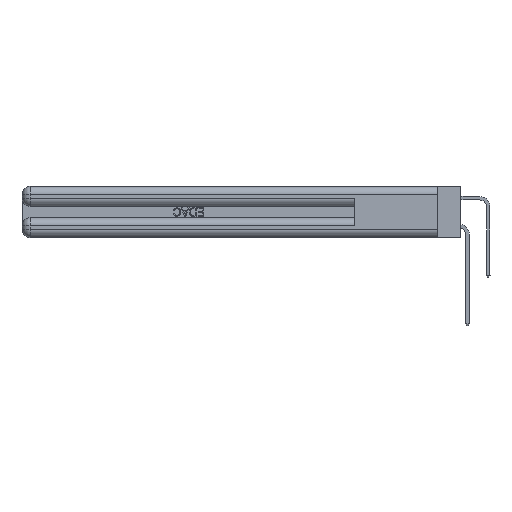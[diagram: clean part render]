
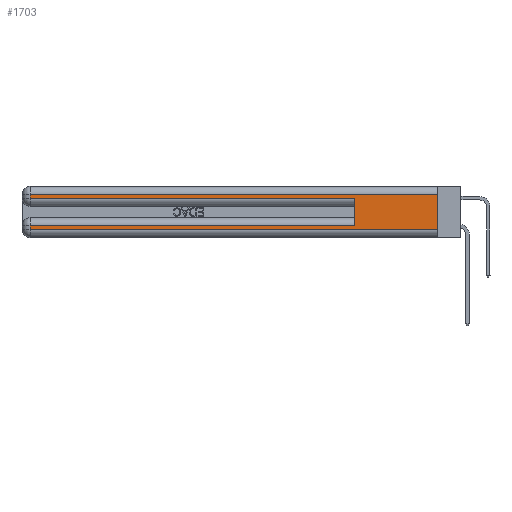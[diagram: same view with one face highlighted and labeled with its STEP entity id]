
A CAD part, left-side view. The second image highlights one B-rep face of the part: STEP entity #1703.
In plain terms, the highlighted planar face has unit normal (-1, 0, 0).
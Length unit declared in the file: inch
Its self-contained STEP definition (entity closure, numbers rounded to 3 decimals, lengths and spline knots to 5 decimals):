
#150 = ORIENTED_EDGE ( 'NONE', *, *, #6819, .T. ) ;
#1618 = EDGE_CURVE ( 'NONE', #8300, #6460, #24683, .T. ) ;
#1642 = ORIENTED_EDGE ( 'NONE', *, *, #17028, .F. ) ;
#1703 = ADVANCED_FACE ( 'NONE', ( #2963 ), #6381, .F. ) ;
#2318 = CARTESIAN_POINT ( 'NONE',  ( 0., 2.94, 0.085 ) ) ;
#2963 = FACE_OUTER_BOUND ( 'NONE', #5443, .T. ) ;
#3741 = AXIS2_PLACEMENT_3D ( 'NONE', #6521, #29088, #16375 ) ;
#3900 = EDGE_CURVE ( 'NONE', #21812, #6460, #6314, .T. ) ;
#5443 = EDGE_LOOP ( 'NONE', ( #24070, #150, #30977, #11613, #1642, #37015, #40231, #34964 ) ) ;
#5729 = DIRECTION ( 'NONE',  ( 0., 1., 0. ) ) ;
#5929 = CARTESIAN_POINT ( 'NONE',  ( 0., 0.6, 0.145 ) ) ;
#6314 = LINE ( 'NONE', #19331, #12859 ) ;
#6381 = PLANE ( 'NONE',  #3741 ) ;
#6460 = VERTEX_POINT ( 'NONE', #27938 ) ;
#6521 = CARTESIAN_POINT ( 'NONE',  ( 0., 0., 0.37 ) ) ;
#6819 = EDGE_CURVE ( 'NONE', #8300, #34189, #9131, .T. ) ;
#8300 = VERTEX_POINT ( 'NONE', #41022 ) ;
#8370 = CARTESIAN_POINT ( 'NONE',  ( 0., 2.94, 0.285 ) ) ;
#8533 = LINE ( 'NONE', #13085, #26160 ) ;
#8828 = VERTEX_POINT ( 'NONE', #28322 ) ;
#9025 = CARTESIAN_POINT ( 'NONE',  ( 0., 0., 0.31 ) ) ;
#9131 = LINE ( 'NONE', #9025, #32344 ) ;
#9233 = VECTOR ( 'NONE', #19887, 39.37008 ) ;
#10529 = DIRECTION ( 'NONE',  ( 0., -1., 0. ) ) ;
#11567 = LINE ( 'NONE', #31318, #31292 ) ;
#11613 = ORIENTED_EDGE ( 'NONE', *, *, #20452, .T. ) ;
#11983 = CARTESIAN_POINT ( 'NONE',  ( 0., 2.94, 0.37 ) ) ;
#12530 = CARTESIAN_POINT ( 'NONE',  ( 0., 2.94, 0.31 ) ) ;
#12859 = VECTOR ( 'NONE', #10529, 39.37008 ) ;
#13085 = CARTESIAN_POINT ( 'NONE',  ( 0., 2.94, 0.37 ) ) ;
#14696 = EDGE_CURVE ( 'NONE', #34189, #15153, #8533, .T. ) ;
#15153 = VERTEX_POINT ( 'NONE', #8370 ) ;
#15453 = VECTOR ( 'NONE', #34585, 39.37008 ) ;
#15518 = DIRECTION ( 'NONE',  ( 0., 0., -1. ) ) ;
#15580 = CARTESIAN_POINT ( 'NONE',  ( 0., 0., 0.37 ) ) ;
#16375 = DIRECTION ( 'NONE',  ( 0., 0., -1. ) ) ;
#17028 = EDGE_CURVE ( 'NONE', #8828, #33573, #39558, .T. ) ;
#19331 = CARTESIAN_POINT ( 'NONE',  ( 0., 0., 0.06 ) ) ;
#19887 = DIRECTION ( 'NONE',  ( 0., 0., 1. ) ) ;
#20452 = EDGE_CURVE ( 'NONE', #15153, #33573, #33755, .T. ) ;
#21812 = VERTEX_POINT ( 'NONE', #30675 ) ;
#23651 = VECTOR ( 'NONE', #41603, 39.37008 ) ;
#24070 = ORIENTED_EDGE ( 'NONE', *, *, #1618, .F. ) ;
#24683 = LINE ( 'NONE', #15580, #23651 ) ;
#26160 = VECTOR ( 'NONE', #15518, 39.37008 ) ;
#26413 = EDGE_CURVE ( 'NONE', #8828, #34741, #11567, .T. ) ;
#27938 = CARTESIAN_POINT ( 'NONE',  ( 0., 0., 0.06 ) ) ;
#28322 = CARTESIAN_POINT ( 'NONE',  ( 0., 0.6, 0.085 ) ) ;
#29088 = DIRECTION ( 'NONE',  ( 1., 0., 0. ) ) ;
#29477 = CARTESIAN_POINT ( 'NONE',  ( 0., 0.6, 0.285 ) ) ;
#30675 = CARTESIAN_POINT ( 'NONE',  ( 0., 2.94, 0.06 ) ) ;
#30977 = ORIENTED_EDGE ( 'NONE', *, *, #14696, .T. ) ;
#31292 = VECTOR ( 'NONE', #5729, 39.37008 ) ;
#31318 = CARTESIAN_POINT ( 'NONE',  ( 0., 0., 0.085 ) ) ;
#31778 = CARTESIAN_POINT ( 'NONE',  ( 0., 0., 0.285 ) ) ;
#32344 = VECTOR ( 'NONE', #41126, 39.37008 ) ;
#33573 = VERTEX_POINT ( 'NONE', #29477 ) ;
#33755 = LINE ( 'NONE', #31778, #41384 ) ;
#34189 = VERTEX_POINT ( 'NONE', #12530 ) ;
#34585 = DIRECTION ( 'NONE',  ( 0., 0., -1. ) ) ;
#34741 = VERTEX_POINT ( 'NONE', #2318 ) ;
#34964 = ORIENTED_EDGE ( 'NONE', *, *, #3900, .T. ) ;
#37015 = ORIENTED_EDGE ( 'NONE', *, *, #26413, .T. ) ;
#37994 = DIRECTION ( 'NONE',  ( 0., -1., 0. ) ) ;
#39558 = LINE ( 'NONE', #5929, #9233 ) ;
#40231 = ORIENTED_EDGE ( 'NONE', *, *, #40342, .T. ) ;
#40342 = EDGE_CURVE ( 'NONE', #34741, #21812, #41271, .T. ) ;
#41022 = CARTESIAN_POINT ( 'NONE',  ( 0., 0., 0.31 ) ) ;
#41126 = DIRECTION ( 'NONE',  ( 0., 1., 0. ) ) ;
#41271 = LINE ( 'NONE', #11983, #15453 ) ;
#41384 = VECTOR ( 'NONE', #37994, 39.37008 ) ;
#41603 = DIRECTION ( 'NONE',  ( 0., 0., -1. ) ) ;
